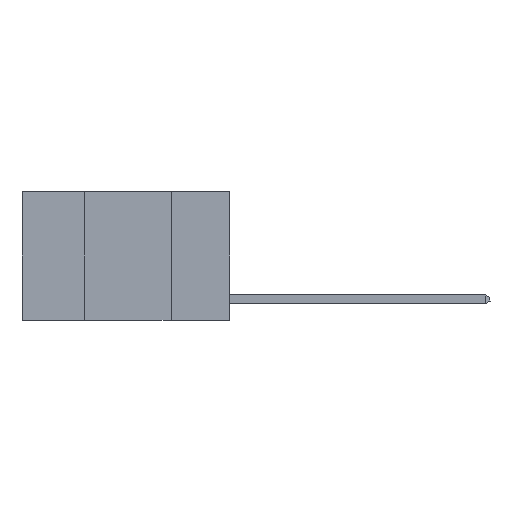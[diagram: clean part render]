
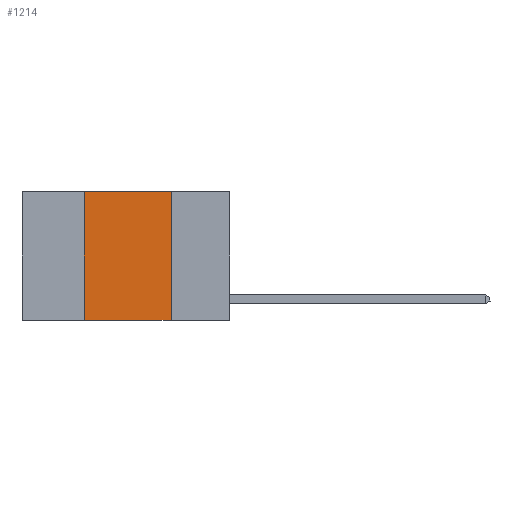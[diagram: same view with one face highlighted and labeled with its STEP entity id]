
A CAD part, left-side view. The second image highlights one B-rep face of the part: STEP entity #1214.
In plain terms, the highlighted planar face has unit normal (-1, 0, 0).
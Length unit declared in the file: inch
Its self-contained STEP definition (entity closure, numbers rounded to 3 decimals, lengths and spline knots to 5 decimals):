
#923 = ORIENTED_EDGE ( 'NONE', *, *, #15800, .F. ) ;
#1214 = ADVANCED_FACE ( 'NONE', ( #7514 ), #16020, .F. ) ;
#2001 = DIRECTION ( 'NONE',  ( 0., -1., 0. ) ) ;
#2002 = ORIENTED_EDGE ( 'NONE', *, *, #6352, .F. ) ;
#4118 = VECTOR ( 'NONE', #4479, 39.37008 ) ;
#4479 = DIRECTION ( 'NONE',  ( 0., -1., 0. ) ) ;
#4931 = VECTOR ( 'NONE', #9914, 39.37008 ) ;
#5034 = EDGE_CURVE ( 'NONE', #17452, #8599, #18563, .T. ) ;
#6081 = CARTESIAN_POINT ( 'NONE',  ( 0., 0.17, 0. ) ) ;
#6352 = EDGE_CURVE ( 'NONE', #13874, #20041, #9736, .T. ) ;
#6441 = CARTESIAN_POINT ( 'NONE',  ( 0., 0.17, 0. ) ) ;
#7306 = LINE ( 'NONE', #19231, #16438 ) ;
#7514 = FACE_OUTER_BOUND ( 'NONE', #11816, .T. ) ;
#8599 = VERTEX_POINT ( 'NONE', #9048 ) ;
#9048 = CARTESIAN_POINT ( 'NONE',  ( 0., 0.17, -0.37 ) ) ;
#9736 = LINE ( 'NONE', #11478, #18251 ) ;
#9821 = ORIENTED_EDGE ( 'NONE', *, *, #5034, .F. ) ;
#9914 = DIRECTION ( 'NONE',  ( 0., 0., -1. ) ) ;
#10906 = CARTESIAN_POINT ( 'NONE',  ( 0., 0.42, -0.37 ) ) ;
#11478 = CARTESIAN_POINT ( 'NONE',  ( 0., 0.42, 0. ) ) ;
#11816 = EDGE_LOOP ( 'NONE', ( #9821, #923, #2002, #14458 ) ) ;
#12628 = EDGE_CURVE ( 'NONE', #13874, #8599, #17852, .T. ) ;
#13874 = VERTEX_POINT ( 'NONE', #10906 ) ;
#14458 = ORIENTED_EDGE ( 'NONE', *, *, #12628, .T. ) ;
#15800 = EDGE_CURVE ( 'NONE', #20041, #17452, #7306, .T. ) ;
#15975 = DIRECTION ( 'NONE',  ( 0., 0., -1. ) ) ;
#15993 = DIRECTION ( 'NONE',  ( 1., 0., 0. ) ) ;
#16020 = PLANE ( 'NONE',  #16382 ) ;
#16248 = CARTESIAN_POINT ( 'NONE',  ( 0., 0.6, 0. ) ) ;
#16382 = AXIS2_PLACEMENT_3D ( 'NONE', #16248, #15993, #15975 ) ;
#16438 = VECTOR ( 'NONE', #2001, 39.37008 ) ;
#16536 = CARTESIAN_POINT ( 'NONE',  ( 0., 0.6, -0.37 ) ) ;
#16611 = DIRECTION ( 'NONE',  ( 0., 0., 1. ) ) ;
#17452 = VERTEX_POINT ( 'NONE', #6081 ) ;
#17852 = LINE ( 'NONE', #16536, #4118 ) ;
#18251 = VECTOR ( 'NONE', #16611, 39.37008 ) ;
#18563 = LINE ( 'NONE', #6441, #4931 ) ;
#19231 = CARTESIAN_POINT ( 'NONE',  ( 0., 0.6, 0. ) ) ;
#19459 = CARTESIAN_POINT ( 'NONE',  ( 0., 0.42, 0. ) ) ;
#20041 = VERTEX_POINT ( 'NONE', #19459 ) ;
